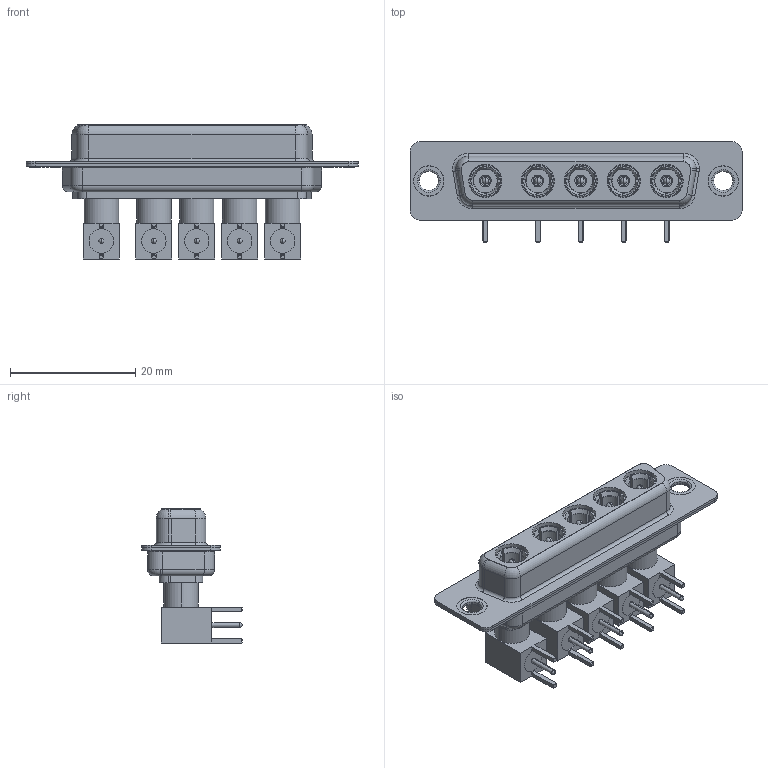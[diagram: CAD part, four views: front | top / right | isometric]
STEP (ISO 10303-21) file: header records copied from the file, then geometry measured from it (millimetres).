
FILE_DESCRIPTION (( 'STEP AP203' ), '1' );
FILE_NAME ('630-5W5-640-7N1.STEP', '2022-06-01T01:42:23', ( '' ), ( '' ), 'SwSTEP 2.0', 'SolidWorks 2020', '' );
FILE_SCHEMA (( 'CONFIG_CONTROL_DESIGN' ));
Length unit declared in the file: millimetre
Products named in the file (16): Co-Ax Plug Assy_RA; 630Combo Shell Rear_25 Contacts; Co-Ax Plug_RA PC Tail; 630Combo Shell Front_25 Contacts; Locking Collar; Insulator RA Pin; Pin_RA; 630Combo Thru Hole Rivet; RA Back Shell; 630Combo Housing_5W5; 630-5W5-640-7N1; Insulator Pin_Straight PC Tail
Assembly tree (40 placements, depth 3):
  630-5W5-640-7N1
    630Combo Housing_5W5
    630Combo Shell Front_25 Contacts
    630Combo Shell Rear_25 Contacts
    630Combo Thru Hole Rivet  x2
    Co-Ax Plug Assy_RA
      Co-Ax Plug_RA PC Tail
      Insulator Pin_Straight PC Tail
      Pin_RA
      Locking Collar
      RA Back Shell
      Insulator RA Pin
    Co-Ax Plug Assy_RA
      Co-Ax Plug_RA PC Tail
      Insulator Pin_Straight PC Tail
      Pin_RA
      Locking Collar
      RA Back Shell
      Insulator RA Pin
    Co-Ax Plug Assy_RA
      Co-Ax Plug_RA PC Tail
      Insulator Pin_Straight PC Tail
      Pin_RA
      Locking Collar
      RA Back Shell
      Insulator RA Pin
    Co-Ax Plug Assy_RA
      Co-Ax Plug_RA PC Tail
      Insulator Pin_Straight PC Tail
      Pin_RA
      Locking Collar
      RA Back Shell
      Insulator RA Pin
    Co-Ax Plug Assy_RA
      Co-Ax Plug_RA PC Tail
      Insulator Pin_Straight PC Tail
      Pin_RA
      Locking Collar
      RA Back Shell
      Insulator RA Pin
Bounding box: 53.05 x 16 x 21.41 mm (x, y, z)
Volume: 4775.3 mm3; surface area: 11649.8 mm2
Topology: 35 solids, 35 shells, 1093 faces, 2608 edges, 1626 vertices
Faces by surface type: cylinder 446, plane 402, cone 125, torus 95, sphere 20, bspline 5
Entity records: 15109 total; most frequent: CARTESIAN_POINT 2528, DIRECTION 2357, ORIENTED_EDGE 2000, EDGE_CURVE 1000, AXIS2_PLACEMENT_3D 960, VERTEX_POINT 628, CIRCLE 492, EDGE_LOOP 482
